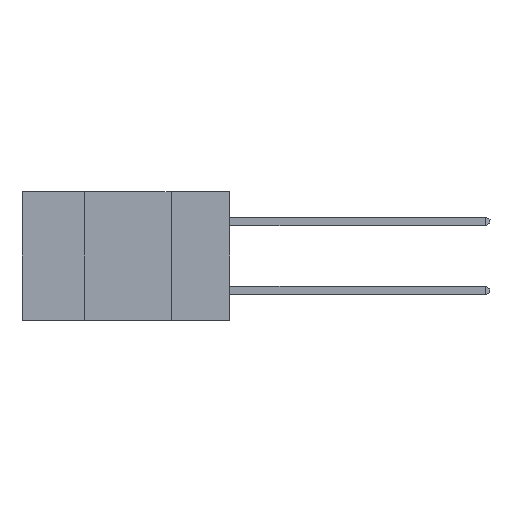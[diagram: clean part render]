
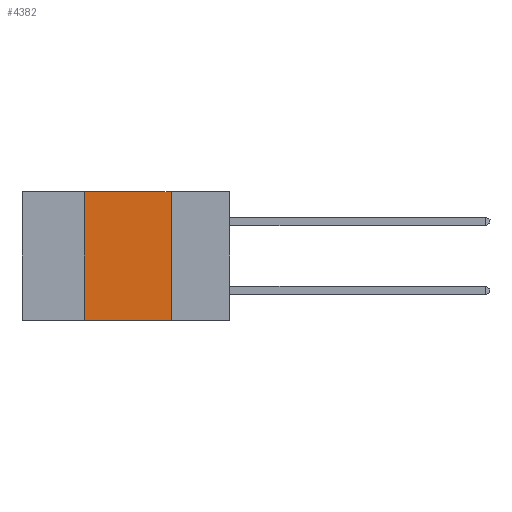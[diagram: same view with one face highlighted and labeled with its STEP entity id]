
A CAD part, left-side view. The second image highlights one B-rep face of the part: STEP entity #4382.
In plain terms, the highlighted planar face has unit normal (-1, 0, 0).
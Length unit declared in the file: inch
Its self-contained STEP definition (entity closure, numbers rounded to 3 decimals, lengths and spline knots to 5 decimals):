
#751 = VERTEX_POINT ( 'NONE', #1157 ) ;
#1157 = CARTESIAN_POINT ( 'NONE',  ( 0., 0.42, 0. ) ) ;
#1164 = ORIENTED_EDGE ( 'NONE', *, *, #3693, .F. ) ;
#1283 = DIRECTION ( 'NONE',  ( 0., 0., -1. ) ) ;
#1420 = CARTESIAN_POINT ( 'NONE',  ( 0., 0.6, 0. ) ) ;
#1840 = LINE ( 'NONE', #3884, #4958 ) ;
#1881 = CARTESIAN_POINT ( 'NONE',  ( 0., 0.42, -0.37 ) ) ;
#2073 = EDGE_CURVE ( 'NONE', #3017, #5385, #2804, .T. ) ;
#2226 = CARTESIAN_POINT ( 'NONE',  ( 0., 0.6, -0.37 ) ) ;
#2804 = LINE ( 'NONE', #4168, #8438 ) ;
#3017 = VERTEX_POINT ( 'NONE', #5805 ) ;
#3159 = DIRECTION ( 'NONE',  ( 0., -1., 0. ) ) ;
#3521 = CARTESIAN_POINT ( 'NONE',  ( 0., 0.42, -0.37 ) ) ;
#3618 = EDGE_CURVE ( 'NONE', #751, #3017, #1840, .T. ) ;
#3668 = VECTOR ( 'NONE', #7787, 39.37008 ) ;
#3693 = EDGE_CURVE ( 'NONE', #3777, #751, #6771, .T. ) ;
#3777 = VERTEX_POINT ( 'NONE', #3521 ) ;
#3884 = CARTESIAN_POINT ( 'NONE',  ( 0., 0.6, 0. ) ) ;
#3950 = EDGE_LOOP ( 'NONE', ( #5180, #7844, #1164, #6892 ) ) ;
#4110 = FACE_OUTER_BOUND ( 'NONE', #3950, .T. ) ;
#4168 = CARTESIAN_POINT ( 'NONE',  ( 0., 0.17, -0.37 ) ) ;
#4199 = DIRECTION ( 'NONE',  ( 1., 0., 0. ) ) ;
#4258 = DIRECTION ( 'NONE',  ( 0., 0., -1. ) ) ;
#4382 = ADVANCED_FACE ( 'NONE', ( #4110 ), #6151, .F. ) ;
#4958 = VECTOR ( 'NONE', #3159, 39.37008 ) ;
#5180 = ORIENTED_EDGE ( 'NONE', *, *, #2073, .F. ) ;
#5385 = VERTEX_POINT ( 'NONE', #5663 ) ;
#5390 = EDGE_CURVE ( 'NONE', #3777, #5385, #8420, .T. ) ;
#5663 = CARTESIAN_POINT ( 'NONE',  ( 0., 0.17, -0.37 ) ) ;
#5805 = CARTESIAN_POINT ( 'NONE',  ( 0., 0.17, 0. ) ) ;
#5973 = DIRECTION ( 'NONE',  ( 0., 0., 1. ) ) ;
#6151 = PLANE ( 'NONE',  #6394 ) ;
#6394 = AXIS2_PLACEMENT_3D ( 'NONE', #1420, #4199, #1283 ) ;
#6771 = LINE ( 'NONE', #1881, #8570 ) ;
#6892 = ORIENTED_EDGE ( 'NONE', *, *, #5390, .T. ) ;
#7787 = DIRECTION ( 'NONE',  ( 0., -1., 0. ) ) ;
#7844 = ORIENTED_EDGE ( 'NONE', *, *, #3618, .F. ) ;
#8420 = LINE ( 'NONE', #2226, #3668 ) ;
#8438 = VECTOR ( 'NONE', #4258, 39.37008 ) ;
#8570 = VECTOR ( 'NONE', #5973, 39.37008 ) ;
